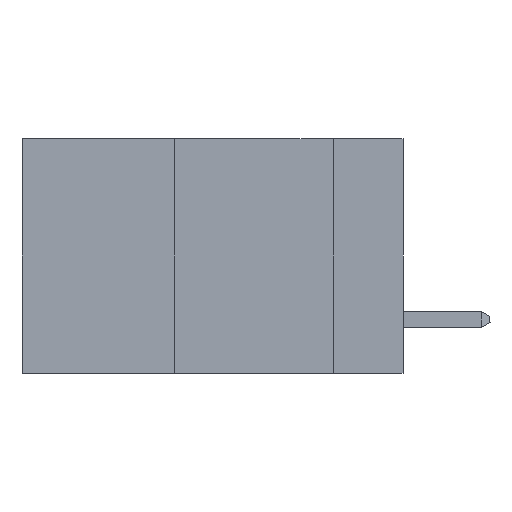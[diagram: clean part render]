
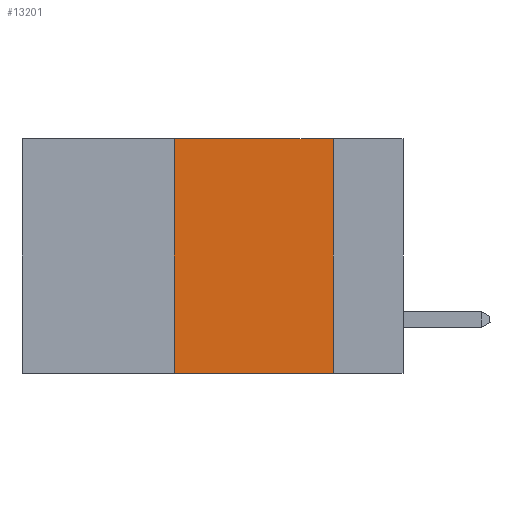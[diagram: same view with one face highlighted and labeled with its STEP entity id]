
A CAD part, left-side view. The second image highlights one B-rep face of the part: STEP entity #13201.
In plain terms, the highlighted planar face has unit normal (-1, 0, 0).
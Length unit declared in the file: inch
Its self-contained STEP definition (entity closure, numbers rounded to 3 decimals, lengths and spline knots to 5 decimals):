
#342 = EDGE_CURVE ( 'NONE', #9860, #13558, #13942, .T. ) ;
#1419 = EDGE_CURVE ( 'NONE', #9860, #12893, #10434, .T. ) ;
#2560 = DIRECTION ( 'NONE',  ( 0., -1., 0. ) ) ;
#2671 = CARTESIAN_POINT ( 'NONE',  ( 0., 0.11, 0. ) ) ;
#2739 = VERTEX_POINT ( 'NONE', #2671 ) ;
#3344 = CARTESIAN_POINT ( 'NONE',  ( 0., 0.36, -0.37 ) ) ;
#3555 = VECTOR ( 'NONE', #10800, 39.37008 ) ;
#3955 = CARTESIAN_POINT ( 'NONE',  ( 0., 0.36, 0. ) ) ;
#4877 = PLANE ( 'NONE',  #7008 ) ;
#6178 = CARTESIAN_POINT ( 'NONE',  ( 0., 0.6, 0. ) ) ;
#6338 = ORIENTED_EDGE ( 'NONE', *, *, #6983, .F. ) ;
#6534 = ORIENTED_EDGE ( 'NONE', *, *, #342, .T. ) ;
#6983 = EDGE_CURVE ( 'NONE', #2739, #13558, #13139, .T. ) ;
#7002 = FACE_OUTER_BOUND ( 'NONE', #14306, .T. ) ;
#7008 = AXIS2_PLACEMENT_3D ( 'NONE', #6178, #15330, #7486 ) ;
#7486 = DIRECTION ( 'NONE',  ( 0., 0., -1. ) ) ;
#7584 = CARTESIAN_POINT ( 'NONE',  ( 0., 0.11, -0.37 ) ) ;
#7996 = CARTESIAN_POINT ( 'NONE',  ( 0., 0.6, 0. ) ) ;
#8546 = CARTESIAN_POINT ( 'NONE',  ( 0., 0.36, 0. ) ) ;
#8781 = CARTESIAN_POINT ( 'NONE',  ( 0., 0.6, -0.37 ) ) ;
#9368 = DIRECTION ( 'NONE',  ( 0., 0., -1. ) ) ;
#9561 = ORIENTED_EDGE ( 'NONE', *, *, #13243, .F. ) ;
#9860 = VERTEX_POINT ( 'NONE', #3344 ) ;
#9875 = DIRECTION ( 'NONE',  ( 0., 0., 1. ) ) ;
#10434 = LINE ( 'NONE', #8546, #12484 ) ;
#10800 = DIRECTION ( 'NONE',  ( 0., -1., 0. ) ) ;
#11080 = ORIENTED_EDGE ( 'NONE', *, *, #1419, .F. ) ;
#11758 = LINE ( 'NONE', #7996, #3555 ) ;
#12484 = VECTOR ( 'NONE', #9875, 39.37008 ) ;
#12893 = VERTEX_POINT ( 'NONE', #3955 ) ;
#13139 = LINE ( 'NONE', #15877, #13347 ) ;
#13201 = ADVANCED_FACE ( 'NONE', ( #7002 ), #4877, .F. ) ;
#13243 = EDGE_CURVE ( 'NONE', #12893, #2739, #11758, .T. ) ;
#13347 = VECTOR ( 'NONE', #9368, 39.37008 ) ;
#13558 = VERTEX_POINT ( 'NONE', #7584 ) ;
#13942 = LINE ( 'NONE', #8781, #14588 ) ;
#14306 = EDGE_LOOP ( 'NONE', ( #6338, #9561, #11080, #6534 ) ) ;
#14588 = VECTOR ( 'NONE', #2560, 39.37008 ) ;
#15330 = DIRECTION ( 'NONE',  ( 1., 0., 0. ) ) ;
#15877 = CARTESIAN_POINT ( 'NONE',  ( 0., 0.11, 0. ) ) ;
